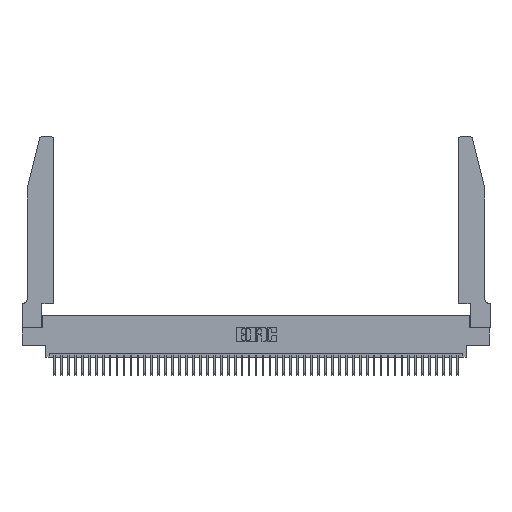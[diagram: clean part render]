
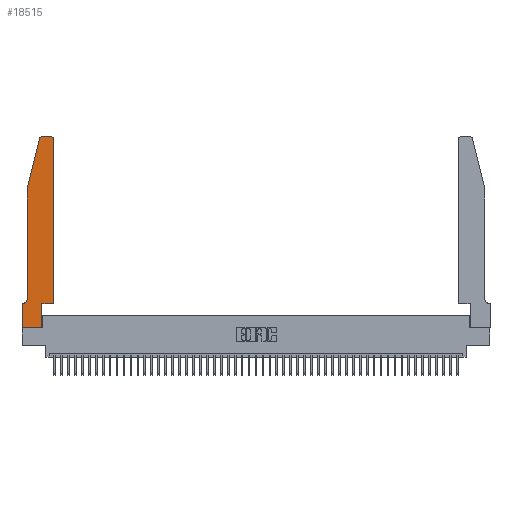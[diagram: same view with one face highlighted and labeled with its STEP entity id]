
A CAD part, top view. The second image highlights one B-rep face of the part: STEP entity #18515.
In plain terms, the highlighted planar face has unit normal (0, 0, 1).
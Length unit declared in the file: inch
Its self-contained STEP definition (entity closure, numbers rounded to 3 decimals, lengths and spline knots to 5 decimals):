
#408 = DIRECTION ( 'NONE',  ( 0., 1., 0. ) ) ;
#901 = CIRCLE ( 'NONE', #8653, 0.03 ) ;
#1119 = CARTESIAN_POINT ( 'NONE',  ( 0., 0.35, 0.37 ) ) ;
#2233 = DIRECTION ( 'NONE',  ( 0., -1., 0. ) ) ;
#2392 = ORIENTED_EDGE ( 'NONE', *, *, #4983, .T. ) ;
#2848 = DIRECTION ( 'NONE',  ( 1., 0., 0. ) ) ;
#3030 = DIRECTION ( 'NONE',  ( 1., 0., 0. ) ) ;
#3133 = DIRECTION ( 'NONE',  ( 0., 1., 0. ) ) ;
#3289 = CARTESIAN_POINT ( 'NONE',  ( 0.2605, 2.75, 0.37 ) ) ;
#3524 = VECTOR ( 'NONE', #12778, 39.37008 ) ;
#3783 = AXIS2_PLACEMENT_3D ( 'NONE', #43361, #12268, #39585 ) ;
#4983 = EDGE_CURVE ( 'NONE', #47742, #17346, #7437, .T. ) ;
#5235 = LINE ( 'NONE', #46010, #19251 ) ;
#5578 = VERTEX_POINT ( 'NONE', #47460 ) ;
#5612 = VERTEX_POINT ( 'NONE', #36818 ) ;
#6416 = CIRCLE ( 'NONE', #33980, 0.03 ) ;
#7055 = DIRECTION ( 'NONE',  ( -1., 0., 0. ) ) ;
#7437 = LINE ( 'NONE', #15219, #39824 ) ;
#8365 = AXIS2_PLACEMENT_3D ( 'NONE', #38179, #34747, #3030 ) ;
#8653 = AXIS2_PLACEMENT_3D ( 'NONE', #22461, #26226, #2848 ) ;
#8686 = EDGE_LOOP ( 'NONE', ( #44492, #46792, #26202, #49753, #18455, #47514, #13261, #10952, #8798, #21557, #2392, #13044 ) ) ;
#8798 = ORIENTED_EDGE ( 'NONE', *, *, #21942, .T. ) ;
#9358 = VERTEX_POINT ( 'NONE', #46980 ) ;
#9955 = LINE ( 'NONE', #43593, #48513 ) ;
#10314 = VERTEX_POINT ( 'NONE', #39498 ) ;
#10952 = ORIENTED_EDGE ( 'NONE', *, *, #20007, .T. ) ;
#12268 = DIRECTION ( 'NONE',  ( 0., 0., -1. ) ) ;
#12439 = EDGE_CURVE ( 'NONE', #38249, #38203, #5235, .T. ) ;
#12778 = DIRECTION ( 'NONE',  ( 1., 0., 0. ) ) ;
#13044 = ORIENTED_EDGE ( 'NONE', *, *, #39280, .T. ) ;
#13261 = ORIENTED_EDGE ( 'NONE', *, *, #38007, .T. ) ;
#14468 = VECTOR ( 'NONE', #42337, 39.37008 ) ;
#14837 = CARTESIAN_POINT ( 'NONE',  ( 0.25487, 2.72718, 0.37 ) ) ;
#15041 = EDGE_CURVE ( 'NONE', #38203, #9358, #42220, .T. ) ;
#15219 = CARTESIAN_POINT ( 'NONE',  ( 0.4505, 0.35, 0.37 ) ) ;
#15679 = CARTESIAN_POINT ( 'NONE',  ( 0.0755, 0.35, 0.37 ) ) ;
#17346 = VERTEX_POINT ( 'NONE', #38450 ) ;
#17460 = LINE ( 'NONE', #37390, #25390 ) ;
#18455 = ORIENTED_EDGE ( 'NONE', *, *, #24553, .T. ) ;
#18515 = ADVANCED_FACE ( 'NONE', ( #47026 ), #38354, .T. ) ;
#18739 = LINE ( 'NONE', #47964, #3524 ) ;
#19251 = VECTOR ( 'NONE', #34385, 39.37008 ) ;
#20007 = EDGE_CURVE ( 'NONE', #5612, #5578, #18739, .T. ) ;
#20696 = CARTESIAN_POINT ( 'NONE',  ( 0.284, 2.75, 0.37 ) ) ;
#21557 = ORIENTED_EDGE ( 'NONE', *, *, #30905, .T. ) ;
#21896 = CARTESIAN_POINT ( 'NONE',  ( 0.4505, 0.35, 0.37 ) ) ;
#21942 = EDGE_CURVE ( 'NONE', #5578, #10314, #9955, .T. ) ;
#22039 = DIRECTION ( 'NONE',  ( 0., 0., 1. ) ) ;
#22195 = DIRECTION ( 'NONE',  ( 1., 0., 0. ) ) ;
#22461 = CARTESIAN_POINT ( 'NONE',  ( 0.284, 2.72, 0.37 ) ) ;
#22600 = EDGE_CURVE ( 'NONE', #45145, #29945, #45353, .T. ) ;
#23022 = CARTESIAN_POINT ( 'NONE',  ( 0.4505, 0.35, 0.37 ) ) ;
#24553 = EDGE_CURVE ( 'NONE', #9358, #45145, #25234, .T. ) ;
#25234 = CIRCLE ( 'NONE', #3783, 0.07 ) ;
#25390 = VECTOR ( 'NONE', #2233, 39.37008 ) ;
#25788 = VECTOR ( 'NONE', #36169, 39.37008 ) ;
#26108 = CARTESIAN_POINT ( 'NONE',  ( 0.4205, 2.75, 0.37 ) ) ;
#26202 = ORIENTED_EDGE ( 'NONE', *, *, #12439, .T. ) ;
#26226 = DIRECTION ( 'NONE',  ( 0., 0., 1. ) ) ;
#27257 = LINE ( 'NONE', #3289, #40692 ) ;
#29279 = EDGE_CURVE ( 'NONE', #43630, #33062, #27257, .T. ) ;
#29472 = CARTESIAN_POINT ( 'NONE',  ( 0.0055, 0.35, 0.37 ) ) ;
#29731 = DIRECTION ( 'NONE',  ( 0., -1., 0. ) ) ;
#29945 = VERTEX_POINT ( 'NONE', #1119 ) ;
#30905 = EDGE_CURVE ( 'NONE', #10314, #47742, #38922, .T. ) ;
#33062 = VERTEX_POINT ( 'NONE', #20696 ) ;
#33980 = AXIS2_PLACEMENT_3D ( 'NONE', #49896, #22039, #22195 ) ;
#34385 = DIRECTION ( 'NONE',  ( -0.239, -0.971, 0. ) ) ;
#34747 = DIRECTION ( 'NONE',  ( 0., 0., 1. ) ) ;
#35503 = VECTOR ( 'NONE', #29731, 39.37008 ) ;
#36169 = DIRECTION ( 'NONE',  ( -1., 0., 0. ) ) ;
#36818 = CARTESIAN_POINT ( 'NONE',  ( 0., 0., 0.37 ) ) ;
#37086 = CARTESIAN_POINT ( 'NONE',  ( 0.0755, 2., 0.37 ) ) ;
#37390 = CARTESIAN_POINT ( 'NONE',  ( 0., 0., 0.37 ) ) ;
#38007 = EDGE_CURVE ( 'NONE', #29945, #5612, #17460, .T. ) ;
#38179 = CARTESIAN_POINT ( 'NONE',  ( 0., 0.35, 0.37 ) ) ;
#38203 = VERTEX_POINT ( 'NONE', #50211 ) ;
#38249 = VERTEX_POINT ( 'NONE', #14837 ) ;
#38354 = PLANE ( 'NONE',  #8365 ) ;
#38450 = CARTESIAN_POINT ( 'NONE',  ( 0.4505, 2.72, 0.37 ) ) ;
#38922 = LINE ( 'NONE', #23022, #14468 ) ;
#39280 = EDGE_CURVE ( 'NONE', #17346, #43630, #6416, .T. ) ;
#39498 = CARTESIAN_POINT ( 'NONE',  ( 0.2865, 0.35, 0.37 ) ) ;
#39585 = DIRECTION ( 'NONE',  ( -1., 0., 0. ) ) ;
#39824 = VECTOR ( 'NONE', #3133, 39.37008 ) ;
#40692 = VECTOR ( 'NONE', #7055, 39.37008 ) ;
#42220 = LINE ( 'NONE', #37086, #35503 ) ;
#42337 = DIRECTION ( 'NONE',  ( 1., 0., 0. ) ) ;
#43361 = CARTESIAN_POINT ( 'NONE',  ( 0.0055, 0.42, 0.37 ) ) ;
#43593 = CARTESIAN_POINT ( 'NONE',  ( 0.2865, 0.35, 0.37 ) ) ;
#43630 = VERTEX_POINT ( 'NONE', #26108 ) ;
#44492 = ORIENTED_EDGE ( 'NONE', *, *, #29279, .T. ) ;
#45145 = VERTEX_POINT ( 'NONE', #29472 ) ;
#45353 = LINE ( 'NONE', #15679, #25788 ) ;
#46010 = CARTESIAN_POINT ( 'NONE',  ( 0.0755, 2., 0.37 ) ) ;
#46792 = ORIENTED_EDGE ( 'NONE', *, *, #48903, .T. ) ;
#46980 = CARTESIAN_POINT ( 'NONE',  ( 0.0755, 0.42, 0.37 ) ) ;
#47026 = FACE_OUTER_BOUND ( 'NONE', #8686, .T. ) ;
#47460 = CARTESIAN_POINT ( 'NONE',  ( 0.2865, 0., 0.37 ) ) ;
#47514 = ORIENTED_EDGE ( 'NONE', *, *, #22600, .T. ) ;
#47742 = VERTEX_POINT ( 'NONE', #21896 ) ;
#47964 = CARTESIAN_POINT ( 'NONE',  ( 0., 0., 0.37 ) ) ;
#48513 = VECTOR ( 'NONE', #408, 39.37008 ) ;
#48903 = EDGE_CURVE ( 'NONE', #33062, #38249, #901, .T. ) ;
#49753 = ORIENTED_EDGE ( 'NONE', *, *, #15041, .T. ) ;
#49896 = CARTESIAN_POINT ( 'NONE',  ( 0.4205, 2.72, 0.37 ) ) ;
#50211 = CARTESIAN_POINT ( 'NONE',  ( 0.0755, 2., 0.37 ) ) ;
